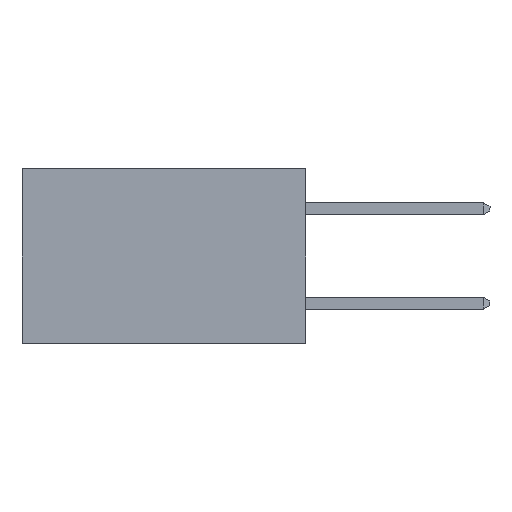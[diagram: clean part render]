
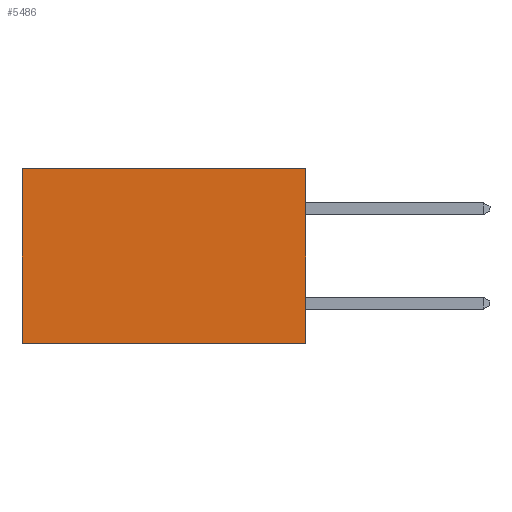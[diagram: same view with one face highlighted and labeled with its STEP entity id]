
A CAD part, left-side view. The second image highlights one B-rep face of the part: STEP entity #5486.
In plain terms, the highlighted planar face has unit normal (-1, 0, 0).
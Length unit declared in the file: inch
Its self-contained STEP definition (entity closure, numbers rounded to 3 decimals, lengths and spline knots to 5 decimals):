
#884 = DIRECTION ( 'NONE',  ( 0., 0., -1. ) ) ;
#1459 = VECTOR ( 'NONE', #8040, 39.37008 ) ;
#1489 = CARTESIAN_POINT ( 'NONE',  ( 0.2615, 0., -0.37 ) ) ;
#1686 = CARTESIAN_POINT ( 'NONE',  ( 0.2615, 0., -0.37 ) ) ;
#1871 = CARTESIAN_POINT ( 'NONE',  ( 0.2615, 0., 0. ) ) ;
#2432 = EDGE_CURVE ( 'NONE', #6374, #7625, #7322, .T. ) ;
#2546 = ORIENTED_EDGE ( 'NONE', *, *, #8955, .T. ) ;
#2793 = ORIENTED_EDGE ( 'NONE', *, *, #5171, .T. ) ;
#3243 = DIRECTION ( 'NONE',  ( 0., 0., -1. ) ) ;
#3412 = DIRECTION ( 'NONE',  ( 1., 0., 0. ) ) ;
#3627 = EDGE_LOOP ( 'NONE', ( #2793, #6703, #3940, #2546 ) ) ;
#3940 = ORIENTED_EDGE ( 'NONE', *, *, #4825, .F. ) ;
#3954 = VERTEX_POINT ( 'NONE', #7565 ) ;
#4493 = AXIS2_PLACEMENT_3D ( 'NONE', #9128, #3412, #6281 ) ;
#4824 = CARTESIAN_POINT ( 'NONE',  ( 0.2615, 0.6, -0.37 ) ) ;
#4825 = EDGE_CURVE ( 'NONE', #6017, #6374, #6205, .T. ) ;
#5171 = EDGE_CURVE ( 'NONE', #3954, #7625, #5875, .T. ) ;
#5206 = CARTESIAN_POINT ( 'NONE',  ( 0.2615, 0.6, -0.37 ) ) ;
#5486 = ADVANCED_FACE ( 'NONE', ( #5576 ), #7743, .F. ) ;
#5576 = FACE_OUTER_BOUND ( 'NONE', #3627, .T. ) ;
#5585 = DIRECTION ( 'NONE',  ( 0., 1., 0. ) ) ;
#5700 = CARTESIAN_POINT ( 'NONE',  ( 0.2615, 0., 0. ) ) ;
#5875 = LINE ( 'NONE', #5206, #9162 ) ;
#6017 = VERTEX_POINT ( 'NONE', #5700 ) ;
#6205 = LINE ( 'NONE', #6873, #7041 ) ;
#6281 = DIRECTION ( 'NONE',  ( 0., 0., -1. ) ) ;
#6374 = VERTEX_POINT ( 'NONE', #1686 ) ;
#6703 = ORIENTED_EDGE ( 'NONE', *, *, #2432, .F. ) ;
#6873 = CARTESIAN_POINT ( 'NONE',  ( 0.2615, 0., -0.37 ) ) ;
#7041 = VECTOR ( 'NONE', #3243, 39.37008 ) ;
#7322 = LINE ( 'NONE', #1489, #1459 ) ;
#7565 = CARTESIAN_POINT ( 'NONE',  ( 0.2615, 0.6, 0. ) ) ;
#7625 = VERTEX_POINT ( 'NONE', #4824 ) ;
#7743 = PLANE ( 'NONE',  #4493 ) ;
#8014 = VECTOR ( 'NONE', #5585, 39.37008 ) ;
#8040 = DIRECTION ( 'NONE',  ( 0., 1., 0. ) ) ;
#8346 = LINE ( 'NONE', #1871, #8014 ) ;
#8955 = EDGE_CURVE ( 'NONE', #6017, #3954, #8346, .T. ) ;
#9128 = CARTESIAN_POINT ( 'NONE',  ( 0.2615, 0., -0.37 ) ) ;
#9162 = VECTOR ( 'NONE', #884, 39.37008 ) ;
